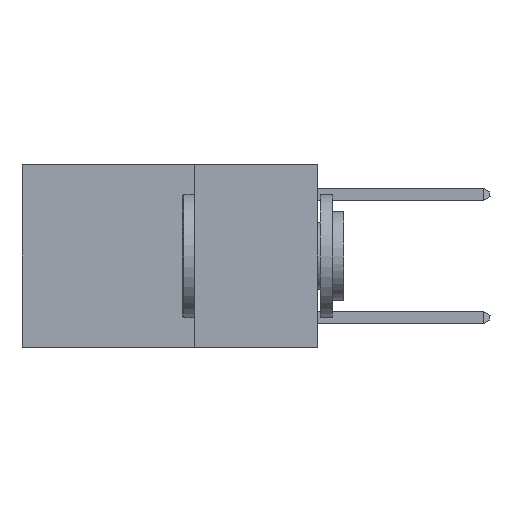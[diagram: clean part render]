
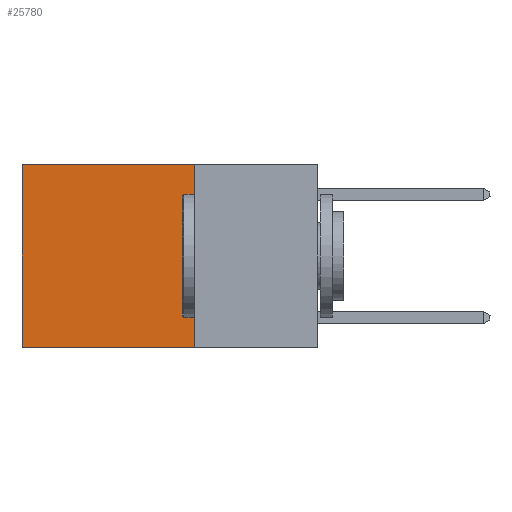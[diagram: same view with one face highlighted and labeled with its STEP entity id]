
A CAD part, left-side view. The second image highlights one B-rep face of the part: STEP entity #25780.
In plain terms, the highlighted planar face has unit normal (-1, 0, 0).
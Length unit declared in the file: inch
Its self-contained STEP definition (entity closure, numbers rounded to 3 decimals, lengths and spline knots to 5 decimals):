
#30 = CARTESIAN_POINT ( 'NONE',  ( 0.2625, 0.6, 0. ) ) ;
#407 = DIRECTION ( 'NONE',  ( 1., 0., 0. ) ) ;
#440 = ORIENTED_EDGE ( 'NONE', *, *, #25693, .T. ) ;
#646 = CARTESIAN_POINT ( 'NONE',  ( 0.2625, 0.25, 0. ) ) ;
#945 = LINE ( 'NONE', #646, #25124 ) ;
#1496 = VECTOR ( 'NONE', #26022, 39.37008 ) ;
#2250 = DIRECTION ( 'NONE',  ( 0., 0., -1. ) ) ;
#2451 = VECTOR ( 'NONE', #23533, 39.37008 ) ;
#2925 = DIRECTION ( 'NONE',  ( 0., 1., 0. ) ) ;
#3573 = ORIENTED_EDGE ( 'NONE', *, *, #17414, .T. ) ;
#4480 = VERTEX_POINT ( 'NONE', #30 ) ;
#6969 = VERTEX_POINT ( 'NONE', #28003 ) ;
#7083 = CARTESIAN_POINT ( 'NONE',  ( 0.2625, 0.25, 0. ) ) ;
#7562 = CARTESIAN_POINT ( 'NONE',  ( 0.2625, 0.25, 0. ) ) ;
#7716 = FACE_OUTER_BOUND ( 'NONE', #25415, .T. ) ;
#7834 = AXIS2_PLACEMENT_3D ( 'NONE', #7562, #407, #23712 ) ;
#9220 = LINE ( 'NONE', #29923, #2451 ) ;
#10153 = PLANE ( 'NONE',  #7834 ) ;
#11987 = CARTESIAN_POINT ( 'NONE',  ( 0.2625, 0.6, 0. ) ) ;
#15500 = VERTEX_POINT ( 'NONE', #7083 ) ;
#16204 = ORIENTED_EDGE ( 'NONE', *, *, #16436, .F. ) ;
#16436 = EDGE_CURVE ( 'NONE', #15500, #16619, #28169, .T. ) ;
#16619 = VERTEX_POINT ( 'NONE', #26792 ) ;
#17414 = EDGE_CURVE ( 'NONE', #15500, #4480, #945, .T. ) ;
#19217 = ORIENTED_EDGE ( 'NONE', *, *, #23228, .F. ) ;
#23228 = EDGE_CURVE ( 'NONE', #16619, #6969, #9220, .T. ) ;
#23533 = DIRECTION ( 'NONE',  ( 0., 1., 0. ) ) ;
#23578 = CARTESIAN_POINT ( 'NONE',  ( 0.2625, 0.25, 0. ) ) ;
#23712 = DIRECTION ( 'NONE',  ( 0., 0., -1. ) ) ;
#25124 = VECTOR ( 'NONE', #2925, 39.37008 ) ;
#25415 = EDGE_LOOP ( 'NONE', ( #440, #19217, #16204, #3573 ) ) ;
#25693 = EDGE_CURVE ( 'NONE', #4480, #6969, #26174, .T. ) ;
#25780 = ADVANCED_FACE ( 'NONE', ( #7716 ), #10153, .F. ) ;
#26022 = DIRECTION ( 'NONE',  ( 0., 0., -1. ) ) ;
#26174 = LINE ( 'NONE', #11987, #1496 ) ;
#26792 = CARTESIAN_POINT ( 'NONE',  ( 0.2625, 0.25, -0.37 ) ) ;
#28003 = CARTESIAN_POINT ( 'NONE',  ( 0.2625, 0.6, -0.37 ) ) ;
#28169 = LINE ( 'NONE', #23578, #28512 ) ;
#28512 = VECTOR ( 'NONE', #2250, 39.37008 ) ;
#29923 = CARTESIAN_POINT ( 'NONE',  ( 0.2625, 0.25, -0.37 ) ) ;
